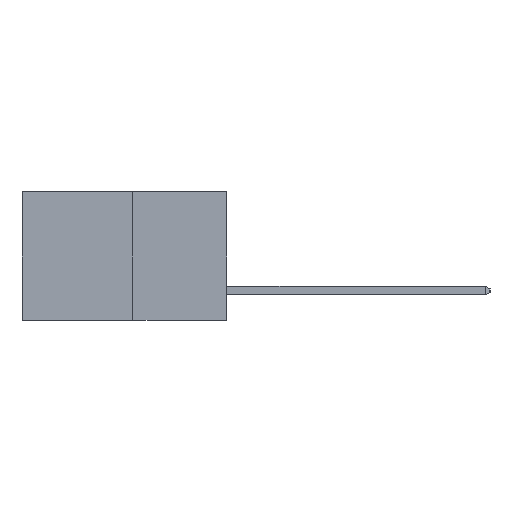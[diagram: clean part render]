
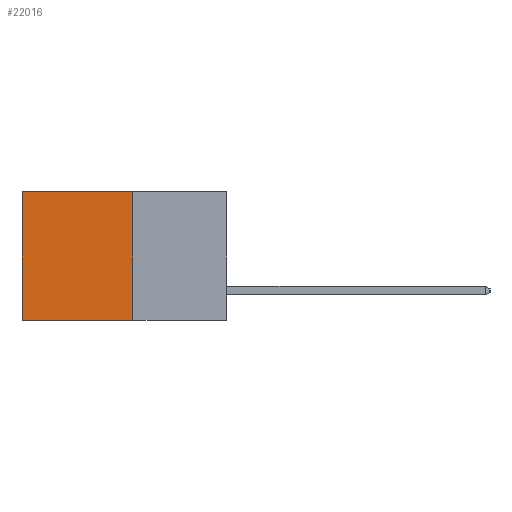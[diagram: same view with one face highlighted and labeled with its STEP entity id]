
A CAD part, left-side view. The second image highlights one B-rep face of the part: STEP entity #22016.
In plain terms, the highlighted planar face has unit normal (-1, 0, 0).
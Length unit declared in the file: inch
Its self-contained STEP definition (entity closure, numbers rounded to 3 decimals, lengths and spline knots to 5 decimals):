
#1579 = VERTEX_POINT ( 'NONE', #12266 ) ;
#2661 = ORIENTED_EDGE ( 'NONE', *, *, #19847, .F. ) ;
#3037 = CARTESIAN_POINT ( 'NONE',  ( 0.277, 0.59, -0.37 ) ) ;
#3420 = LINE ( 'NONE', #4115, #29861 ) ;
#4115 = CARTESIAN_POINT ( 'NONE',  ( 0.277, 0.59, -0.37 ) ) ;
#4959 = EDGE_CURVE ( 'NONE', #21393, #1579, #23611, .T. ) ;
#6125 = DIRECTION ( 'NONE',  ( 1., 0., 0. ) ) ;
#6693 = ORIENTED_EDGE ( 'NONE', *, *, #18089, .F. ) ;
#7931 = VERTEX_POINT ( 'NONE', #3037 ) ;
#10296 = DIRECTION ( 'NONE',  ( 0., 1., 0. ) ) ;
#10632 = ORIENTED_EDGE ( 'NONE', *, *, #4959, .T. ) ;
#12151 = CARTESIAN_POINT ( 'NONE',  ( 0.277, 0.27, 0. ) ) ;
#12266 = CARTESIAN_POINT ( 'NONE',  ( 0.277, 0.59, 0. ) ) ;
#14850 = EDGE_CURVE ( 'NONE', #1579, #7931, #3420, .T. ) ;
#15481 = LINE ( 'NONE', #27700, #16271 ) ;
#16271 = VECTOR ( 'NONE', #10296, 39.37008 ) ;
#16385 = CARTESIAN_POINT ( 'NONE',  ( 0.277, 0.27, 0. ) ) ;
#18056 = FACE_OUTER_BOUND ( 'NONE', #21920, .T. ) ;
#18089 = EDGE_CURVE ( 'NONE', #21244, #7931, #15481, .T. ) ;
#19655 = DIRECTION ( 'NONE',  ( 0., 1., 0. ) ) ;
#19844 = AXIS2_PLACEMENT_3D ( 'NONE', #21016, #6125, #23535 ) ;
#19847 = EDGE_CURVE ( 'NONE', #21393, #21244, #22307, .T. ) ;
#20526 = DIRECTION ( 'NONE',  ( 0., 0., -1. ) ) ;
#21016 = CARTESIAN_POINT ( 'NONE',  ( 0.277, 0.27, -0.37 ) ) ;
#21244 = VERTEX_POINT ( 'NONE', #28242 ) ;
#21393 = VERTEX_POINT ( 'NONE', #16385 ) ;
#21920 = EDGE_LOOP ( 'NONE', ( #27165, #6693, #2661, #10632 ) ) ;
#22016 = ADVANCED_FACE ( 'NONE', ( #18056 ), #30907, .F. ) ;
#22307 = LINE ( 'NONE', #27926, #27373 ) ;
#23535 = DIRECTION ( 'NONE',  ( 0., 0., -1. ) ) ;
#23611 = LINE ( 'NONE', #12151, #29419 ) ;
#27165 = ORIENTED_EDGE ( 'NONE', *, *, #14850, .T. ) ;
#27373 = VECTOR ( 'NONE', #20526, 39.37008 ) ;
#27700 = CARTESIAN_POINT ( 'NONE',  ( 0.277, 0.27, -0.37 ) ) ;
#27926 = CARTESIAN_POINT ( 'NONE',  ( 0.277, 0.27, -0.37 ) ) ;
#28242 = CARTESIAN_POINT ( 'NONE',  ( 0.277, 0.27, -0.37 ) ) ;
#29419 = VECTOR ( 'NONE', #19655, 39.37008 ) ;
#29861 = VECTOR ( 'NONE', #30718, 39.37008 ) ;
#30718 = DIRECTION ( 'NONE',  ( 0., 0., -1. ) ) ;
#30907 = PLANE ( 'NONE',  #19844 ) ;
